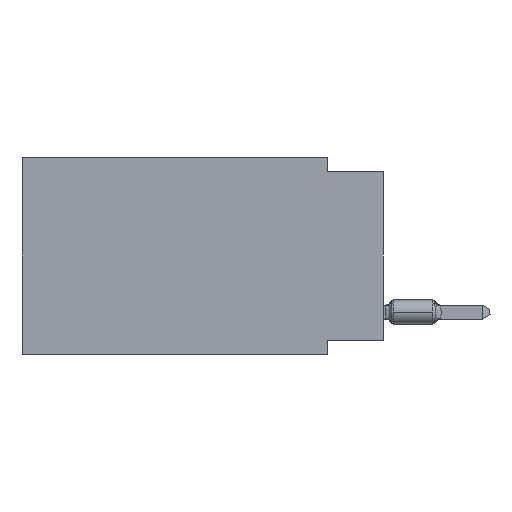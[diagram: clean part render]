
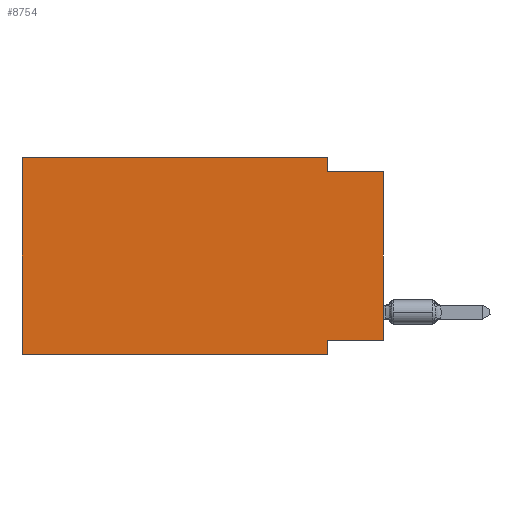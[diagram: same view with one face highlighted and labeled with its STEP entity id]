
A CAD part, left-side view. The second image highlights one B-rep face of the part: STEP entity #8754.
In plain terms, the highlighted planar face has unit normal (-1, 0, 0).
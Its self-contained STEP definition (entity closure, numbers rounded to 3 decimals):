
#441 = VERTEX_POINT ( 'NONE', #24111 ) ;
#1985 = DIRECTION ( 'NONE',  ( 1., 0., 0. ) ) ;
#3598 = CARTESIAN_POINT ( 'NONE',  ( 0., 16.383, 0. ) ) ;
#5861 = EDGE_CURVE ( 'NONE', #24233, #25175, #31803, .T. ) ;
#6391 = EDGE_CURVE ( 'NONE', #24233, #25122, #9295, .T. ) ;
#6832 = VECTOR ( 'NONE', #43478, 1000. ) ;
#6853 = LINE ( 'NONE', #10726, #37198 ) ;
#7118 = DIRECTION ( 'NONE',  ( 0., 0., -1. ) ) ;
#8754 = ADVANCED_FACE ( 'NONE', ( #29676 ), #21659, .F. ) ;
#8824 = ORIENTED_EDGE ( 'NONE', *, *, #28389, .T. ) ;
#9295 = LINE ( 'NONE', #25092, #26920 ) ;
#10181 = EDGE_CURVE ( 'NONE', #441, #44356, #6853, .T. ) ;
#10726 = CARTESIAN_POINT ( 'NONE',  ( 0., 0., -8.255 ) ) ;
#10829 = LINE ( 'NONE', #39085, #6832 ) ;
#11025 = DIRECTION ( 'NONE',  ( 0., 0., -1. ) ) ;
#14406 = CARTESIAN_POINT ( 'NONE',  ( 0., 2.54, 0. ) ) ;
#14911 = LINE ( 'NONE', #30978, #25043 ) ;
#15263 = CARTESIAN_POINT ( 'NONE',  ( 0., 2.54, -0.635 ) ) ;
#15581 = CARTESIAN_POINT ( 'NONE',  ( 0., 16.383, 0. ) ) ;
#17224 = AXIS2_PLACEMENT_3D ( 'NONE', #33804, #1985, #25787 ) ;
#19619 = VERTEX_POINT ( 'NONE', #15263 ) ;
#19642 = DIRECTION ( 'NONE',  ( 0., -1., 0. ) ) ;
#21659 = PLANE ( 'NONE',  #17224 ) ;
#22652 = DIRECTION ( 'NONE',  ( 0., 1., 0. ) ) ;
#23274 = CARTESIAN_POINT ( 'NONE',  ( 0., 0., -0.635 ) ) ;
#24111 = CARTESIAN_POINT ( 'NONE',  ( 0., 0., -8.255 ) ) ;
#24233 = VERTEX_POINT ( 'NONE', #48966 ) ;
#24659 = VECTOR ( 'NONE', #31052, 1000. ) ;
#25043 = VECTOR ( 'NONE', #11025, 1000. ) ;
#25092 = CARTESIAN_POINT ( 'NONE',  ( 0., 16.383, -8.89 ) ) ;
#25122 = VERTEX_POINT ( 'NONE', #40326 ) ;
#25175 = VERTEX_POINT ( 'NONE', #15581 ) ;
#25549 = EDGE_CURVE ( 'NONE', #19619, #29578, #49959, .T. ) ;
#25787 = DIRECTION ( 'NONE',  ( 0., 0., -1. ) ) ;
#26920 = VECTOR ( 'NONE', #40907, 1000. ) ;
#27027 = ORIENTED_EDGE ( 'NONE', *, *, #38963, .F. ) ;
#28389 = EDGE_CURVE ( 'NONE', #441, #29578, #10829, .T. ) ;
#28460 = CARTESIAN_POINT ( 'NONE',  ( 0., 2.54, -8.255 ) ) ;
#29578 = VERTEX_POINT ( 'NONE', #23274 ) ;
#29676 = FACE_OUTER_BOUND ( 'NONE', #44941, .T. ) ;
#30643 = VECTOR ( 'NONE', #19642, 1000. ) ;
#30754 = ORIENTED_EDGE ( 'NONE', *, *, #32673, .F. ) ;
#30978 = CARTESIAN_POINT ( 'NONE',  ( 0., 2.54, -8.89 ) ) ;
#31052 = DIRECTION ( 'NONE',  ( 0., -1., 0. ) ) ;
#31259 = CARTESIAN_POINT ( 'NONE',  ( 0., 16.383, 0. ) ) ;
#31803 = LINE ( 'NONE', #31259, #33543 ) ;
#32673 = EDGE_CURVE ( 'NONE', #25175, #34508, #34406, .T. ) ;
#33221 = ORIENTED_EDGE ( 'NONE', *, *, #10181, .F. ) ;
#33543 = VECTOR ( 'NONE', #47319, 1000. ) ;
#33804 = CARTESIAN_POINT ( 'NONE',  ( 0., 16.383, 0. ) ) ;
#34406 = LINE ( 'NONE', #3598, #30643 ) ;
#34508 = VERTEX_POINT ( 'NONE', #14406 ) ;
#37198 = VECTOR ( 'NONE', #22652, 1000. ) ;
#37968 = ORIENTED_EDGE ( 'NONE', *, *, #6391, .T. ) ;
#38963 = EDGE_CURVE ( 'NONE', #44356, #25122, #14911, .T. ) ;
#39085 = CARTESIAN_POINT ( 'NONE',  ( 0., 0., 0. ) ) ;
#40326 = CARTESIAN_POINT ( 'NONE',  ( 0., 2.54, -8.89 ) ) ;
#40907 = DIRECTION ( 'NONE',  ( 0., -1., 0. ) ) ;
#43319 = ORIENTED_EDGE ( 'NONE', *, *, #25549, .F. ) ;
#43478 = DIRECTION ( 'NONE',  ( 0., 0., 1. ) ) ;
#44356 = VERTEX_POINT ( 'NONE', #28460 ) ;
#44941 = EDGE_LOOP ( 'NONE', ( #8824, #43319, #49975, #30754, #46175, #37968, #27027, #33221 ) ) ;
#45835 = CARTESIAN_POINT ( 'NONE',  ( 0., 0., -0.635 ) ) ;
#45980 = LINE ( 'NONE', #50351, #50660 ) ;
#46175 = ORIENTED_EDGE ( 'NONE', *, *, #5861, .F. ) ;
#47319 = DIRECTION ( 'NONE',  ( 0., 0., 1. ) ) ;
#48966 = CARTESIAN_POINT ( 'NONE',  ( 0., 16.383, -8.89 ) ) ;
#49644 = EDGE_CURVE ( 'NONE', #34508, #19619, #45980, .T. ) ;
#49959 = LINE ( 'NONE', #45835, #24659 ) ;
#49975 = ORIENTED_EDGE ( 'NONE', *, *, #49644, .F. ) ;
#50351 = CARTESIAN_POINT ( 'NONE',  ( 0., 2.54, 0. ) ) ;
#50660 = VECTOR ( 'NONE', #7118, 1000. ) ;
